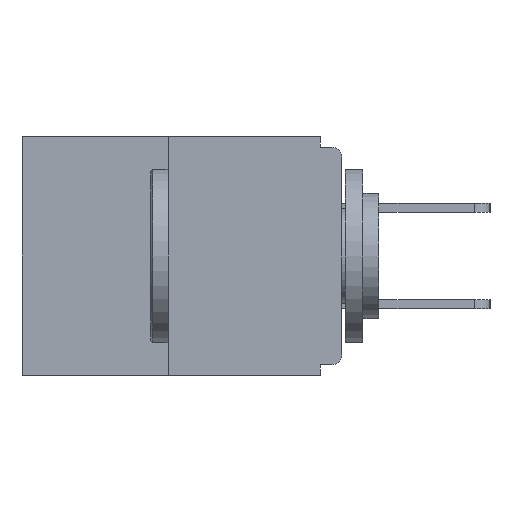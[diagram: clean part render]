
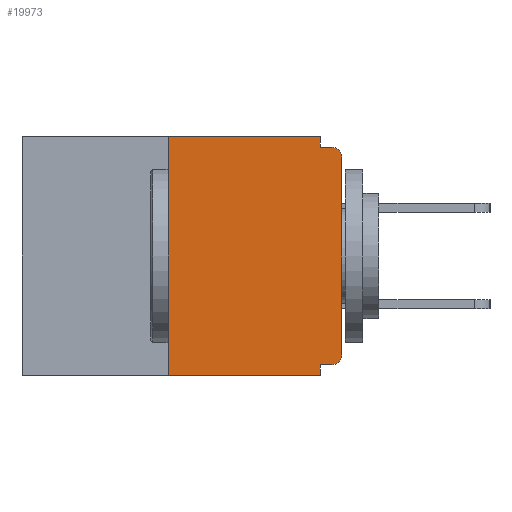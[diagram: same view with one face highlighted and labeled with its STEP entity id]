
A CAD part, left-side view. The second image highlights one B-rep face of the part: STEP entity #19973.
In plain terms, the highlighted planar face has unit normal (-1, 0, 0).
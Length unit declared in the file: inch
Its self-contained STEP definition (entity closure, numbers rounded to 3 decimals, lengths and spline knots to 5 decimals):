
#646 = LINE ( 'NONE', #14450, #19430 ) ;
#689 = CIRCLE ( 'NONE', #4392, 0.015 ) ;
#728 = ORIENTED_EDGE ( 'NONE', *, *, #798, .T. ) ;
#798 = EDGE_CURVE ( 'NONE', #4695, #9502, #13215, .T. ) ;
#991 = LINE ( 'NONE', #20199, #18285 ) ;
#1608 = ORIENTED_EDGE ( 'NONE', *, *, #4195, .T. ) ;
#1704 = DIRECTION ( 'NONE',  ( 0., 0., -1. ) ) ;
#1716 = ORIENTED_EDGE ( 'NONE', *, *, #20486, .F. ) ;
#1914 = CARTESIAN_POINT ( 'NONE',  ( 0., 0., 0. ) ) ;
#2096 = ORIENTED_EDGE ( 'NONE', *, *, #20408, .F. ) ;
#2184 = DIRECTION ( 'NONE',  ( -1., 0., 0. ) ) ;
#2287 = LINE ( 'NONE', #18715, #10449 ) ;
#2448 = CARTESIAN_POINT ( 'NONE',  ( 0., 0.25, -0.343 ) ) ;
#2670 = VECTOR ( 'NONE', #13645, 39.37008 ) ;
#2856 = CARTESIAN_POINT ( 'NONE',  ( 0., 0.015, -0.015 ) ) ;
#3130 = CARTESIAN_POINT ( 'NONE',  ( 0., 0.25, 0. ) ) ;
#3707 = CARTESIAN_POINT ( 'NONE',  ( 0., 0.015, -0.03 ) ) ;
#4195 = EDGE_CURVE ( 'NONE', #13699, #8442, #2287, .T. ) ;
#4282 = EDGE_CURVE ( 'NONE', #9502, #6941, #14419, .T. ) ;
#4392 = AXIS2_PLACEMENT_3D ( 'NONE', #5241, #8356, #9796 ) ;
#4695 = VERTEX_POINT ( 'NONE', #15703 ) ;
#5241 = CARTESIAN_POINT ( 'NONE',  ( 0., 0.015, -0.313 ) ) ;
#5704 = ORIENTED_EDGE ( 'NONE', *, *, #4282, .T. ) ;
#6128 = DIRECTION ( 'NONE',  ( 0., -1., 0. ) ) ;
#6941 = VERTEX_POINT ( 'NONE', #2856 ) ;
#7574 = CARTESIAN_POINT ( 'NONE',  ( 0., 0.46, 0. ) ) ;
#8356 = DIRECTION ( 'NONE',  ( -1., 0., 0. ) ) ;
#8442 = VERTEX_POINT ( 'NONE', #10933 ) ;
#9017 = PLANE ( 'NONE',  #14458 ) ;
#9164 = ORIENTED_EDGE ( 'NONE', *, *, #11205, .T. ) ;
#9264 = DIRECTION ( 'NONE',  ( 0., -1., 0. ) ) ;
#9291 = VERTEX_POINT ( 'NONE', #19072 ) ;
#9502 = VERTEX_POINT ( 'NONE', #15239 ) ;
#9796 = DIRECTION ( 'NONE',  ( 0., 0., -1. ) ) ;
#9878 = CARTESIAN_POINT ( 'NONE',  ( 0., 0., -0.015 ) ) ;
#10449 = VECTOR ( 'NONE', #9264, 39.37008 ) ;
#10594 = DIRECTION ( 'NONE',  ( 0., 0., -1. ) ) ;
#10765 = EDGE_CURVE ( 'NONE', #12390, #9291, #19447, .T. ) ;
#10883 = FACE_OUTER_BOUND ( 'NONE', #13897, .T. ) ;
#10933 = CARTESIAN_POINT ( 'NONE',  ( 0., 0.031, -0.343 ) ) ;
#10952 = CARTESIAN_POINT ( 'NONE',  ( 0., 0.46, 0. ) ) ;
#11205 = EDGE_CURVE ( 'NONE', #12390, #4695, #689, .T. ) ;
#11482 = ORIENTED_EDGE ( 'NONE', *, *, #18884, .F. ) ;
#11596 = CARTESIAN_POINT ( 'NONE',  ( 0., 0.031, 0. ) ) ;
#11905 = ORIENTED_EDGE ( 'NONE', *, *, #16684, .F. ) ;
#12389 = VECTOR ( 'NONE', #6128, 39.37008 ) ;
#12390 = VERTEX_POINT ( 'NONE', #17735 ) ;
#12883 = DIRECTION ( 'NONE',  ( 0., 0., -1. ) ) ;
#13215 = LINE ( 'NONE', #1914, #18372 ) ;
#13645 = DIRECTION ( 'NONE',  ( 0., 1., 0. ) ) ;
#13699 = VERTEX_POINT ( 'NONE', #2448 ) ;
#13703 = LINE ( 'NONE', #14414, #16880 ) ;
#13774 = CARTESIAN_POINT ( 'NONE',  ( 0., 0., -0.328 ) ) ;
#13897 = EDGE_LOOP ( 'NONE', ( #2096, #1716, #1608, #19304, #16445, #9164, #728, #5704, #11482, #11905 ) ) ;
#14414 = CARTESIAN_POINT ( 'NONE',  ( 0., 0.031, -0.343 ) ) ;
#14419 = CIRCLE ( 'NONE', #19454, 0.015 ) ;
#14450 = CARTESIAN_POINT ( 'NONE',  ( 0., 0.031, 0. ) ) ;
#14458 = AXIS2_PLACEMENT_3D ( 'NONE', #7574, #18526, #10594 ) ;
#15239 = CARTESIAN_POINT ( 'NONE',  ( 0., 0., -0.03 ) ) ;
#15659 = VERTEX_POINT ( 'NONE', #3130 ) ;
#15703 = CARTESIAN_POINT ( 'NONE',  ( 0., 0., -0.313 ) ) ;
#16022 = DIRECTION ( 'NONE',  ( 0., -1., 0. ) ) ;
#16068 = LINE ( 'NONE', #10952, #12389 ) ;
#16445 = ORIENTED_EDGE ( 'NONE', *, *, #10765, .F. ) ;
#16684 = EDGE_CURVE ( 'NONE', #20143, #19140, #646, .T. ) ;
#16880 = VECTOR ( 'NONE', #12883, 39.37008 ) ;
#17717 = DIRECTION ( 'NONE',  ( 0., 0., 1. ) ) ;
#17735 = CARTESIAN_POINT ( 'NONE',  ( 0., 0.015, -0.328 ) ) ;
#18285 = VECTOR ( 'NONE', #19076, 39.37008 ) ;
#18367 = EDGE_CURVE ( 'NONE', #9291, #8442, #13703, .T. ) ;
#18372 = VECTOR ( 'NONE', #17717, 39.37008 ) ;
#18526 = DIRECTION ( 'NONE',  ( 1., 0., 0. ) ) ;
#18579 = VECTOR ( 'NONE', #16022, 39.37008 ) ;
#18715 = CARTESIAN_POINT ( 'NONE',  ( 0., 0.46, -0.343 ) ) ;
#18884 = EDGE_CURVE ( 'NONE', #19140, #6941, #19577, .T. ) ;
#19072 = CARTESIAN_POINT ( 'NONE',  ( 0., 0.031, -0.328 ) ) ;
#19076 = DIRECTION ( 'NONE',  ( 0., 0., 1. ) ) ;
#19140 = VERTEX_POINT ( 'NONE', #19834 ) ;
#19304 = ORIENTED_EDGE ( 'NONE', *, *, #18367, .F. ) ;
#19369 = DIRECTION ( 'NONE',  ( 0., 0., -1. ) ) ;
#19430 = VECTOR ( 'NONE', #1704, 39.37008 ) ;
#19447 = LINE ( 'NONE', #13774, #2670 ) ;
#19454 = AXIS2_PLACEMENT_3D ( 'NONE', #3707, #2184, #19369 ) ;
#19577 = LINE ( 'NONE', #9878, #18579 ) ;
#19834 = CARTESIAN_POINT ( 'NONE',  ( 0., 0.031, -0.015 ) ) ;
#19973 = ADVANCED_FACE ( 'NONE', ( #10883 ), #9017, .F. ) ;
#20143 = VERTEX_POINT ( 'NONE', #11596 ) ;
#20199 = CARTESIAN_POINT ( 'NONE',  ( 0., 0.25, 0. ) ) ;
#20408 = EDGE_CURVE ( 'NONE', #15659, #20143, #16068, .T. ) ;
#20486 = EDGE_CURVE ( 'NONE', #13699, #15659, #991, .T. ) ;
